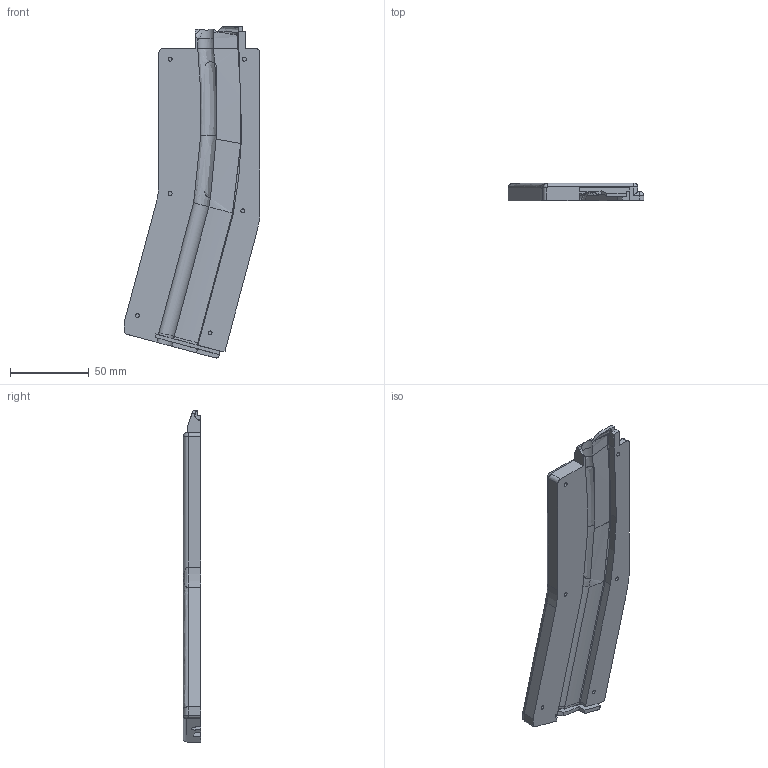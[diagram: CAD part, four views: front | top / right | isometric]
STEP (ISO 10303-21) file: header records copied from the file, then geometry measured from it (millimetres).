
FILE_DESCRIPTION(/* description */ (''),/* implementation_level */ '2;1');
FILE_NAME(/* name */ 'Left Body 25.step',/* time_stamp */ '2021-06-10T14:12:30-07:00',/* author */ (''),/* organization */ (''),/* preprocessor_version */ 'ST-DEVELOPER v18.1',/* originating_system */ 'Autodesk Translation Framework v10.9.0.1377',/* authorisation */ '');
FILE_SCHEMA (('AUTOMOTIVE_DESIGN { 1 0 10303 214 3 1 1 }'));
Length unit declared in the file: millimetre
Products named in the file (1): BodyL
Bounding box: 86 x 11 x 210.15 mm (x, y, z)
Volume: 107003.4 mm3; surface area: 34028.8 mm2
Topology: 1 solids, 1 shells, 180 faces, 461 edges, 282 vertices
Faces by surface type: plane 71, bspline 60, cylinder 45, torus 2, sphere 2
Full cylindrical faces by diameter (mm): 2.5 x6
Entity records: 7952 total; most frequent: CARTESIAN_POINT 3936, ORIENTED_EDGE 908, DIRECTION 705, EDGE_CURVE 454, VERTEX_POINT 282, AXIS2_PLACEMENT_3D 259, LINE 187, VECTOR 187
